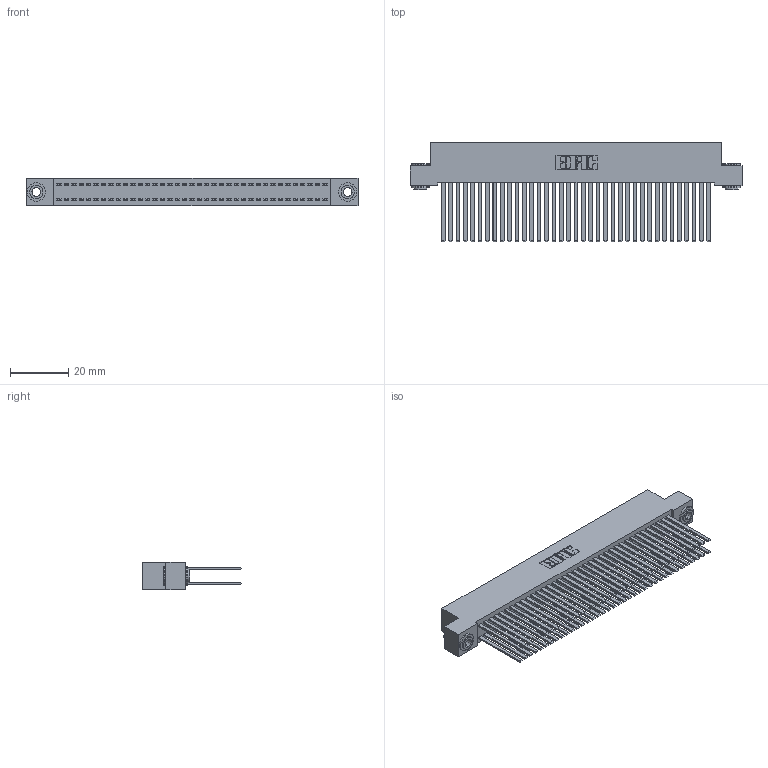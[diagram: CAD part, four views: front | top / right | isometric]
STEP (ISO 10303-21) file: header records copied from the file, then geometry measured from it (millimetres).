
FILE_DESCRIPTION (( 'STEP AP203' ), '1' );
FILE_NAME ('392-074-544-203.STEP', '2018-08-18T00:53:36', ( '' ), ( '' ), 'SwSTEP 2.0', 'SolidWorks 2016', '' );
FILE_SCHEMA (( 'CONFIG_CONTROL_DESIGN' ));
Length unit declared in the file: inch
Products named in the file (4): 342-250-002_345-250-002-102; 392-074-544-203; 342 Part_.156 TH; 345-292-001_345-293-144
Assembly tree (77 placements, depth 2):
  392-074-544-203
    342 Part_.156 TH
    345-292-001_345-293-144  x74
    342-250-002_345-250-002-102  x2
Bounding box: 114.3 x 34.3 x 9.4 mm (x, y, z)
Volume: 11306.3 mm3; surface area: 21367.5 mm2
Topology: 77 solids, 77 shells, 3552 faces, 10513 edges, 6906 vertices
Faces by surface type: plane 2444, cylinder 1100, cone 8
Entity records: 24784 total; most frequent: CARTESIAN_POINT 4085, ORIENTED_EDGE 4014, DIRECTION 3529, EDGE_CURVE 2007, VECTOR 1859, LINE 1859, VERTEX_POINT 1334, AXIS2_PLACEMENT_3D 835
